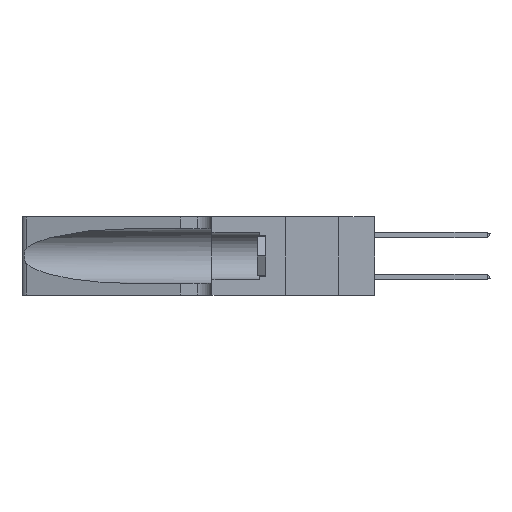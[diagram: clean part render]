
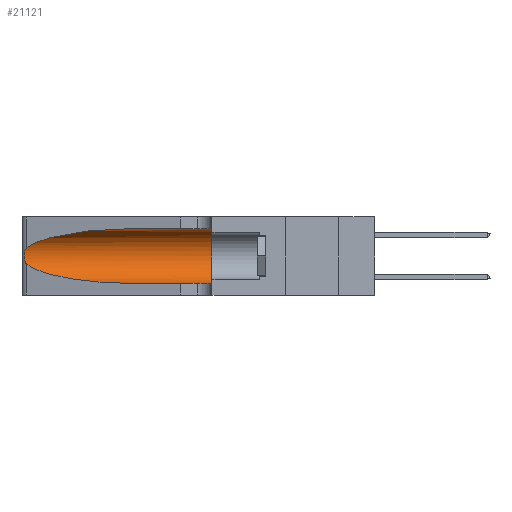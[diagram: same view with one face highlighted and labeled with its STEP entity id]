
A CAD part, left-side view. The second image highlights one B-rep face of the part: STEP entity #21121.
In plain terms, the highlighted cylindrical face has radius 3.308 mm (diameter 6.617 mm), a partial arc.
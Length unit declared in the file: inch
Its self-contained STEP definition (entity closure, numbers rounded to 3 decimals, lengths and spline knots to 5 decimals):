
#234 = CARTESIAN_POINT ( 'NONE',  ( 0.25555, 1.22994, 0.2215 ) ) ;
#399 = CARTESIAN_POINT ( 'NONE',  ( 0.25639, 1.23186, 0.15144 ) ) ;
#3438 = ORIENTED_EDGE ( 'NONE', *, *, #9002, .T. ) ;
#3877 = CARTESIAN_POINT ( 'NONE',  ( 0.18966, 0.96281, 0.05475 ) ) ;
#3941 = CARTESIAN_POINT ( 'NONE',  ( 0.25487, 1.22718, 0.22369 ) ) ;
#4111 = CARTESIAN_POINT ( 'NONE',  ( 0.25487, 1.22718, 0.14631 ) ) ;
#4183 = ORIENTED_EDGE ( 'NONE', *, *, #25940, .T. ) ;
#5445 = VECTOR ( 'NONE', #38444, 39.37008 ) ;
#7358 = CARTESIAN_POINT ( 'NONE',  ( 0.2373, 1.15595, 0.08982 ) ) ;
#7577 = CARTESIAN_POINT ( 'NONE',  ( 0.25639, 1.23184, 0.21858 ) ) ;
#7748 = VERTEX_POINT ( 'NONE', #21298 ) ;
#7801 = ORIENTED_EDGE ( 'NONE', *, *, #27867, .T. ) ;
#9002 = EDGE_CURVE ( 'NONE', #9781, #7748, #32148, .T. ) ;
#9026 = DIRECTION ( 'NONE',  ( 0., 1., 0. ) ) ;
#9702 = EDGE_CURVE ( 'NONE', #15979, #37479, #22175, .T. ) ;
#9781 = VERTEX_POINT ( 'NONE', #29471 ) ;
#10215 = DIRECTION ( 'NONE',  ( 0., 0., -1. ) ) ;
#11254 = CARTESIAN_POINT ( 'NONE',  ( 0.25854, 1.2359, 0.20912 ) ) ;
#12076 = CIRCLE ( 'NONE', #21619, 0.13025 ) ;
#12096 =( BOUNDED_CURVE ( )  B_SPLINE_CURVE ( 3, ( #25289, #7358, #3877, #29017 ),
 .UNSPECIFIED., .F., .T. ) 
 B_SPLINE_CURVE_WITH_KNOTS ( ( 4, 4 ),
 ( 3.44316, 4.71239 ),
 .UNSPECIFIED. ) 
 CURVE ( )  GEOMETRIC_REPRESENTATION_ITEM ( )  RATIONAL_B_SPLINE_CURVE ( ( 1., 0.87, 0.87, 1. ) ) 
 REPRESENTATION_ITEM ( '' )  );
#12605 = VECTOR ( 'NONE', #25610, 39.37008 ) ;
#13261 = VERTEX_POINT ( 'NONE', #31765 ) ;
#13561 = CARTESIAN_POINT ( 'NONE',  ( 0.1305, 1.61858, 0.31525 ) ) ;
#13685 = EDGE_CURVE ( 'NONE', #13261, #37479, #12076, .T. ) ;
#14882 = CARTESIAN_POINT ( 'NONE',  ( 0.26075, 1.23896, 0.19203 ) ) ;
#15738 = CYLINDRICAL_SURFACE ( 'NONE', #36306, 0.13025 ) ;
#15979 = VERTEX_POINT ( 'NONE', #35677 ) ;
#17688 = EDGE_CURVE ( 'NONE', #20935, #13261, #24597, .T. ) ;
#18517 = CARTESIAN_POINT ( 'NONE',  ( 0.26017, 1.23833, 0.17102 ) ) ;
#20935 = VERTEX_POINT ( 'NONE', #27184 ) ;
#21121 = ADVANCED_FACE ( 'NONE', ( #28606 ), #15738, .F. ) ;
#21298 = CARTESIAN_POINT ( 'NONE',  ( 0.25487, 1.22718, 0.14631 ) ) ;
#21619 = AXIS2_PLACEMENT_3D ( 'NONE', #30496, #9026, #34024 ) ;
#22104 = CARTESIAN_POINT ( 'NONE',  ( 0.25789, 1.23486, 0.15765 ) ) ;
#22175 = LINE ( 'NONE', #32580, #12605 ) ;
#23464 = CARTESIAN_POINT ( 'NONE',  ( 0.25487, 1.22718, 0.22369 ) ) ;
#23685 = ORIENTED_EDGE ( 'NONE', *, *, #9702, .T. ) ;
#24597 = LINE ( 'NONE', #13561, #5445 ) ;
#25289 = CARTESIAN_POINT ( 'NONE',  ( 0.25487, 1.22718, 0.14631 ) ) ;
#25610 = DIRECTION ( 'NONE',  ( 0., -1., 0. ) ) ;
#25661 = CARTESIAN_POINT ( 'NONE',  ( 0.25555, 1.22993, 0.14849 ) ) ;
#25940 = EDGE_CURVE ( 'NONE', #20935, #9781, #28725, .T. ) ;
#26872 = CARTESIAN_POINT ( 'NONE',  ( 0.1305, 0.72297, 0.31525 ) ) ;
#27184 = CARTESIAN_POINT ( 'NONE',  ( 0.1305, 0.72297, 0.31525 ) ) ;
#27867 = EDGE_CURVE ( 'NONE', #7748, #15979, #12096, .T. ) ;
#28091 = DIRECTION ( 'NONE',  ( 0., -1., 0. ) ) ;
#28606 = FACE_OUTER_BOUND ( 'NONE', #45902, .T. ) ;
#28725 =( BOUNDED_CURVE ( )  B_SPLINE_CURVE ( 3, ( #26872, #30427, #44653, #23464 ),
 .UNSPECIFIED., .F., .T. ) 
 B_SPLINE_CURVE_WITH_KNOTS ( ( 4, 4 ),
 ( 1.5708, 2.84003 ),
 .UNSPECIFIED. ) 
 CURVE ( )  GEOMETRIC_REPRESENTATION_ITEM ( )  RATIONAL_B_SPLINE_CURVE ( ( 1., 0.87, 0.87, 1. ) ) 
 REPRESENTATION_ITEM ( '' )  );
#29017 = CARTESIAN_POINT ( 'NONE',  ( 0.1305, 0.72297, 0.05475 ) ) ;
#29471 = CARTESIAN_POINT ( 'NONE',  ( 0.25487, 1.22718, 0.22369 ) ) ;
#30427 = CARTESIAN_POINT ( 'NONE',  ( 0.18966, 0.96281, 0.31525 ) ) ;
#30496 = CARTESIAN_POINT ( 'NONE',  ( 0.1305, 0.35, 0.185 ) ) ;
#31639 = CARTESIAN_POINT ( 'NONE',  ( 0.1305, 1.61858, 0.185 ) ) ;
#31765 = CARTESIAN_POINT ( 'NONE',  ( 0.1305, 0.35, 0.31525 ) ) ;
#32148 = B_SPLINE_CURVE_WITH_KNOTS ( 'NONE', 3,
 ( #3941, #234, #7577, #32636, #11254, #36186, #14882, #39729, #18517, #43310, #22104, #399, #25661, #4111 ),
 .UNSPECIFIED., .F., .F.,
 ( 4, 2, 2, 2, 2, 2, 4 ),
 ( 0., 0.00027, 0.00053, 0.00107, 0.0016, 0.00187, 0.00214 ),
 .UNSPECIFIED. ) ;
#32387 = CARTESIAN_POINT ( 'NONE',  ( 0.1305, 0.35, 0.05475 ) ) ;
#32580 = CARTESIAN_POINT ( 'NONE',  ( 0.1305, 1.61858, 0.05475 ) ) ;
#32636 = CARTESIAN_POINT ( 'NONE',  ( 0.25787, 1.23484, 0.2124 ) ) ;
#34024 = DIRECTION ( 'NONE',  ( 0., 0., 1. ) ) ;
#35677 = CARTESIAN_POINT ( 'NONE',  ( 0.1305, 0.72297, 0.05475 ) ) ;
#36186 = CARTESIAN_POINT ( 'NONE',  ( 0.26018, 1.23835, 0.19895 ) ) ;
#36306 = AXIS2_PLACEMENT_3D ( 'NONE', #31639, #28091, #10215 ) ;
#37479 = VERTEX_POINT ( 'NONE', #32387 ) ;
#38444 = DIRECTION ( 'NONE',  ( 0., -1., 0. ) ) ;
#39729 = CARTESIAN_POINT ( 'NONE',  ( 0.26075, 1.23896, 0.178 ) ) ;
#43310 = CARTESIAN_POINT ( 'NONE',  ( 0.25856, 1.23593, 0.16098 ) ) ;
#43506 = ORIENTED_EDGE ( 'NONE', *, *, #13685, .F. ) ;
#44653 = CARTESIAN_POINT ( 'NONE',  ( 0.2373, 1.15595, 0.28018 ) ) ;
#45902 = EDGE_LOOP ( 'NONE', ( #4183, #3438, #7801, #23685, #43506, #46107 ) ) ;
#46107 = ORIENTED_EDGE ( 'NONE', *, *, #17688, .F. ) ;
